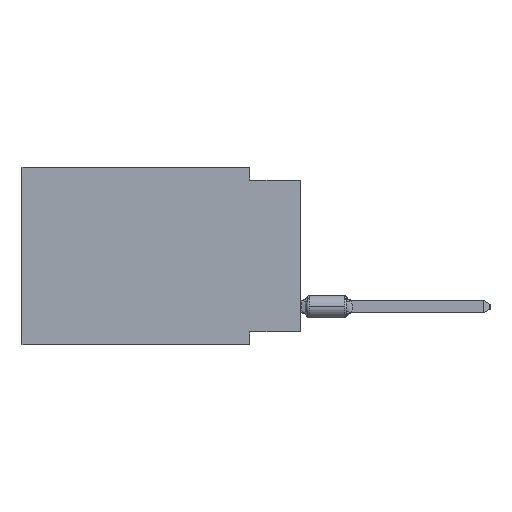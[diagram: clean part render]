
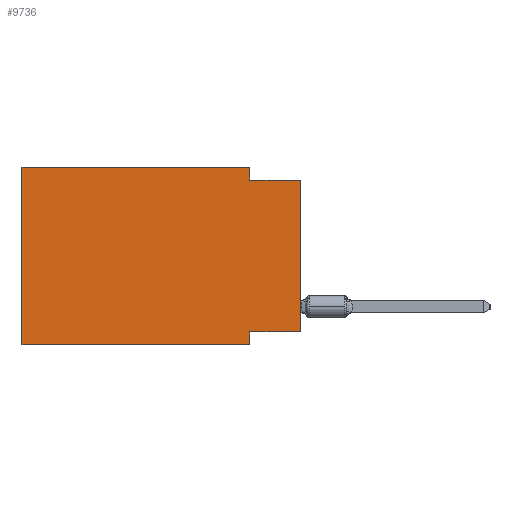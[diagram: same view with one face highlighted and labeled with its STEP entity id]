
A CAD part, left-side view. The second image highlights one B-rep face of the part: STEP entity #9736.
In plain terms, the highlighted planar face has unit normal (-1, 0, 0).
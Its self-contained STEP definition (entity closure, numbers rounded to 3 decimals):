
#508 = LINE ( 'NONE', #10920, #23188 ) ;
#634 = VECTOR ( 'NONE', #10852, 1000. ) ;
#1042 = LINE ( 'NONE', #22571, #17810 ) ;
#1106 = ORIENTED_EDGE ( 'NONE', *, *, #12291, .F. ) ;
#1235 = EDGE_CURVE ( 'NONE', #2431, #11507, #22838, .T. ) ;
#1611 = CARTESIAN_POINT ( 'NONE',  ( 0., 0., -8.255 ) ) ;
#1766 = CARTESIAN_POINT ( 'NONE',  ( 0., 2.54, -8.255 ) ) ;
#1798 = EDGE_CURVE ( 'NONE', #16006, #2431, #16411, .T. ) ;
#1984 = VERTEX_POINT ( 'NONE', #1766 ) ;
#2431 = VERTEX_POINT ( 'NONE', #6132 ) ;
#2911 = CARTESIAN_POINT ( 'NONE',  ( 0., 0., 0. ) ) ;
#3034 = EDGE_CURVE ( 'NONE', #6858, #15876, #508, .T. ) ;
#3037 = DIRECTION ( 'NONE',  ( 0., 0., -1. ) ) ;
#4382 = ORIENTED_EDGE ( 'NONE', *, *, #13410, .F. ) ;
#4708 = DIRECTION ( 'NONE',  ( 0., 0., 1. ) ) ;
#5156 = CARTESIAN_POINT ( 'NONE',  ( 0., 2.54, -8.89 ) ) ;
#5338 = VECTOR ( 'NONE', #17294, 1000. ) ;
#6132 = CARTESIAN_POINT ( 'NONE',  ( 0., 2.54, -0.635 ) ) ;
#6858 = VERTEX_POINT ( 'NONE', #22649 ) ;
#6955 = CARTESIAN_POINT ( 'NONE',  ( 0., 0., -8.255 ) ) ;
#8354 = VERTEX_POINT ( 'NONE', #11480 ) ;
#8538 = AXIS2_PLACEMENT_3D ( 'NONE', #24313, #16615, #3037 ) ;
#8543 = ORIENTED_EDGE ( 'NONE', *, *, #1798, .F. ) ;
#8585 = ORIENTED_EDGE ( 'NONE', *, *, #9848, .T. ) ;
#8834 = ORIENTED_EDGE ( 'NONE', *, *, #9029, .F. ) ;
#9029 = EDGE_CURVE ( 'NONE', #1984, #15876, #15186, .T. ) ;
#9346 = VECTOR ( 'NONE', #22417, 1000. ) ;
#9736 = ADVANCED_FACE ( 'NONE', ( #20932 ), #14519, .F. ) ;
#9848 = EDGE_CURVE ( 'NONE', #15332, #11507, #20803, .T. ) ;
#10134 = VECTOR ( 'NONE', #14880, 1000. ) ;
#10852 = DIRECTION ( 'NONE',  ( 0., 0., 1. ) ) ;
#10920 = CARTESIAN_POINT ( 'NONE',  ( 0., 13.97, -8.89 ) ) ;
#11068 = ORIENTED_EDGE ( 'NONE', *, *, #12969, .F. ) ;
#11480 = CARTESIAN_POINT ( 'NONE',  ( 0., 13.97, 0. ) ) ;
#11507 = VERTEX_POINT ( 'NONE', #22728 ) ;
#12114 = ORIENTED_EDGE ( 'NONE', *, *, #3034, .T. ) ;
#12291 = EDGE_CURVE ( 'NONE', #8354, #16006, #19491, .T. ) ;
#12495 = CARTESIAN_POINT ( 'NONE',  ( 0., 2.54, 0. ) ) ;
#12770 = ORIENTED_EDGE ( 'NONE', *, *, #1235, .F. ) ;
#12969 = EDGE_CURVE ( 'NONE', #6858, #8354, #1042, .T. ) ;
#13410 = EDGE_CURVE ( 'NONE', #15332, #1984, #19508, .T. ) ;
#13947 = CARTESIAN_POINT ( 'NONE',  ( 0., 2.54, -8.89 ) ) ;
#14519 = PLANE ( 'NONE',  #8538 ) ;
#14880 = DIRECTION ( 'NONE',  ( 0., -1., 0. ) ) ;
#14967 = DIRECTION ( 'NONE',  ( 0., -1., 0. ) ) ;
#15186 = LINE ( 'NONE', #5156, #19785 ) ;
#15332 = VERTEX_POINT ( 'NONE', #6955 ) ;
#15686 = VECTOR ( 'NONE', #21451, 1000. ) ;
#15876 = VERTEX_POINT ( 'NONE', #13947 ) ;
#16006 = VERTEX_POINT ( 'NONE', #12495 ) ;
#16411 = LINE ( 'NONE', #24102, #9346 ) ;
#16615 = DIRECTION ( 'NONE',  ( 1., 0., 0. ) ) ;
#17294 = DIRECTION ( 'NONE',  ( 0., 1., 0. ) ) ;
#17810 = VECTOR ( 'NONE', #4708, 1000. ) ;
#19491 = LINE ( 'NONE', #23133, #15686 ) ;
#19508 = LINE ( 'NONE', #1611, #5338 ) ;
#19785 = VECTOR ( 'NONE', #23385, 1000. ) ;
#20803 = LINE ( 'NONE', #2911, #634 ) ;
#20932 = FACE_OUTER_BOUND ( 'NONE', #25645, .T. ) ;
#21451 = DIRECTION ( 'NONE',  ( 0., -1., 0. ) ) ;
#22417 = DIRECTION ( 'NONE',  ( 0., 0., -1. ) ) ;
#22571 = CARTESIAN_POINT ( 'NONE',  ( 0., 13.97, 0. ) ) ;
#22649 = CARTESIAN_POINT ( 'NONE',  ( 0., 13.97, -8.89 ) ) ;
#22728 = CARTESIAN_POINT ( 'NONE',  ( 0., 0., -0.635 ) ) ;
#22838 = LINE ( 'NONE', #24805, #10134 ) ;
#23133 = CARTESIAN_POINT ( 'NONE',  ( 0., 13.97, 0. ) ) ;
#23188 = VECTOR ( 'NONE', #14967, 1000. ) ;
#23385 = DIRECTION ( 'NONE',  ( 0., 0., -1. ) ) ;
#24102 = CARTESIAN_POINT ( 'NONE',  ( 0., 2.54, 0. ) ) ;
#24313 = CARTESIAN_POINT ( 'NONE',  ( 0., 13.97, 0. ) ) ;
#24805 = CARTESIAN_POINT ( 'NONE',  ( 0., 0., -0.635 ) ) ;
#25645 = EDGE_LOOP ( 'NONE', ( #8585, #12770, #8543, #1106, #11068, #12114, #8834, #4382 ) ) ;
